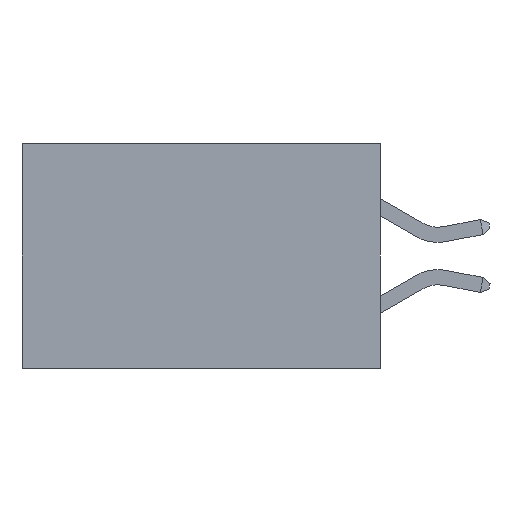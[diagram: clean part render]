
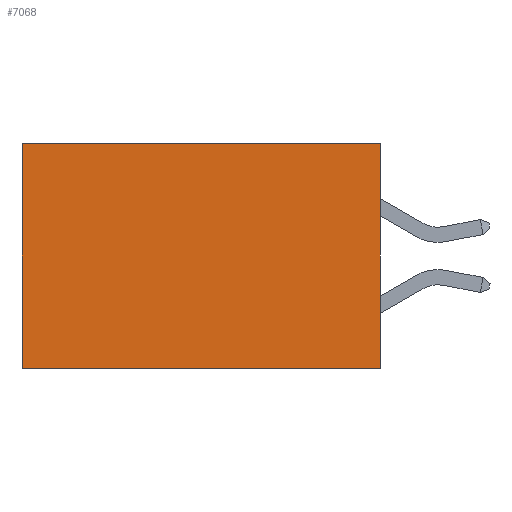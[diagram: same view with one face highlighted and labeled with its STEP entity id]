
A CAD part, left-side view. The second image highlights one B-rep face of the part: STEP entity #7068.
In plain terms, the highlighted planar face has unit normal (-1, 0, 0).
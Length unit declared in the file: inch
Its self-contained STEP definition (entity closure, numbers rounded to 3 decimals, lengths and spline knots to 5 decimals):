
#612 = EDGE_CURVE ( 'NONE', #9037, #4656, #9285, .T. ) ;
#931 = EDGE_CURVE ( 'NONE', #7297, #4883, #4370, .T. ) ;
#958 = AXIS2_PLACEMENT_3D ( 'NONE', #6092, #6044, #6020 ) ;
#1043 = VECTOR ( 'NONE', #6009, 39.37008 ) ;
#1321 = CARTESIAN_POINT ( 'NONE',  ( 0.277, 0.59, -0.37 ) ) ;
#1592 = CARTESIAN_POINT ( 'NONE',  ( 0.277, 0., -0.37 ) ) ;
#1705 = LINE ( 'NONE', #7691, #3464 ) ;
#2315 = EDGE_LOOP ( 'NONE', ( #4538, #4688, #4693, #4713 ) ) ;
#2563 = CARTESIAN_POINT ( 'NONE',  ( 0.277, 0., -0.37 ) ) ;
#2713 = LINE ( 'NONE', #4184, #4783 ) ;
#3464 = VECTOR ( 'NONE', #7173, 39.37008 ) ;
#3602 = EDGE_CURVE ( 'NONE', #7297, #9037, #1705, .T. ) ;
#3632 = VECTOR ( 'NONE', #3774, 39.37008 ) ;
#3774 = DIRECTION ( 'NONE',  ( 0., 0., -1. ) ) ;
#3959 = CARTESIAN_POINT ( 'NONE',  ( 0.277, 0.59, 0. ) ) ;
#4177 = DIRECTION ( 'NONE',  ( 0., 1., 0. ) ) ;
#4184 = CARTESIAN_POINT ( 'NONE',  ( 0.277, 0., -0.37 ) ) ;
#4370 = LINE ( 'NONE', #1592, #1043 ) ;
#4538 = ORIENTED_EDGE ( 'NONE', *, *, #612, .T. ) ;
#4656 = VERTEX_POINT ( 'NONE', #1321 ) ;
#4688 = ORIENTED_EDGE ( 'NONE', *, *, #7715, .F. ) ;
#4693 = ORIENTED_EDGE ( 'NONE', *, *, #931, .F. ) ;
#4713 = ORIENTED_EDGE ( 'NONE', *, *, #3602, .T. ) ;
#4783 = VECTOR ( 'NONE', #4177, 39.37008 ) ;
#4883 = VERTEX_POINT ( 'NONE', #2563 ) ;
#5013 = PLANE ( 'NONE',  #958 ) ;
#5471 = CARTESIAN_POINT ( 'NONE',  ( 0.277, 0., 0. ) ) ;
#6009 = DIRECTION ( 'NONE',  ( 0., 0., -1. ) ) ;
#6020 = DIRECTION ( 'NONE',  ( 0., 0., -1. ) ) ;
#6044 = DIRECTION ( 'NONE',  ( 1., 0., 0. ) ) ;
#6092 = CARTESIAN_POINT ( 'NONE',  ( 0.277, 0., -0.37 ) ) ;
#7068 = ADVANCED_FACE ( 'NONE', ( #8729 ), #5013, .F. ) ;
#7173 = DIRECTION ( 'NONE',  ( 0., 1., 0. ) ) ;
#7297 = VERTEX_POINT ( 'NONE', #5471 ) ;
#7558 = CARTESIAN_POINT ( 'NONE',  ( 0.277, 0.59, -0.37 ) ) ;
#7691 = CARTESIAN_POINT ( 'NONE',  ( 0.277, 0., 0. ) ) ;
#7715 = EDGE_CURVE ( 'NONE', #4883, #4656, #2713, .T. ) ;
#8729 = FACE_OUTER_BOUND ( 'NONE', #2315, .T. ) ;
#9037 = VERTEX_POINT ( 'NONE', #3959 ) ;
#9285 = LINE ( 'NONE', #7558, #3632 ) ;
